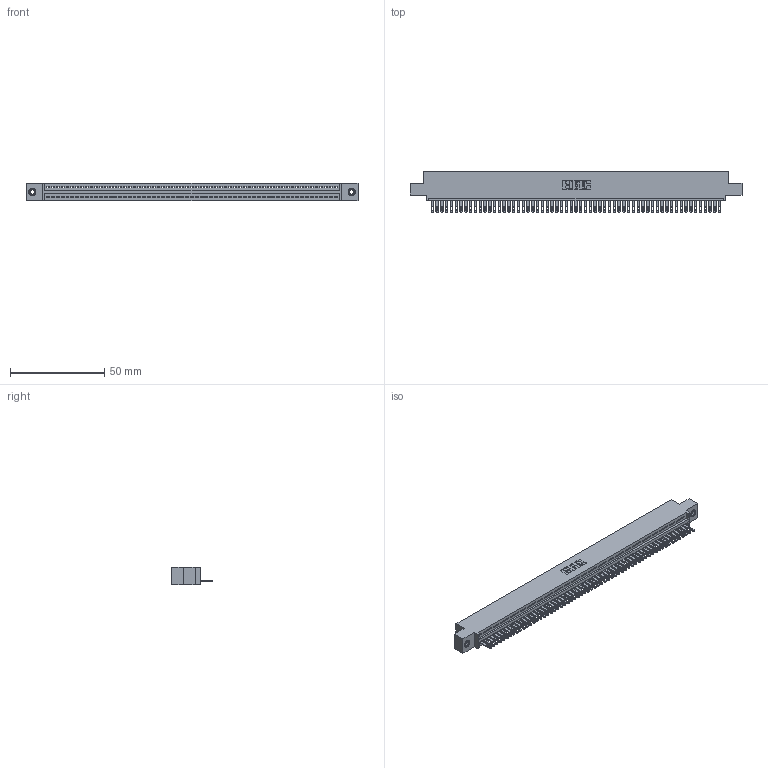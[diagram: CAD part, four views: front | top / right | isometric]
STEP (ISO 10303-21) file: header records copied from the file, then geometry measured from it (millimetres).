
FILE_DESCRIPTION (( 'STEP AP203' ), '1' );
FILE_NAME ('895-061-500-408.STEP', '2020-09-28T06:13:03', ( '' ), ( '' ), 'SwSTEP 2.0', 'SolidWorks 2020', '' );
FILE_SCHEMA (( 'CONFIG_CONTROL_DESIGN' ));
Length unit declared in the file: inch
Products named in the file (4): 345-292-001_345-293-100; 345-250-001_345-250-003-102; 895-061-500-408; 845 Part_0.110 Offset - 0.156 Dia-TI
Assembly tree (64 placements, depth 2):
  895-061-500-408
    845 Part_0.110 Offset - 0.156 Dia-TI
    345-292-001_345-293-100  x61
    345-250-001_345-250-003-102  x2
Bounding box: 176.15 x 21.51 x 9.4 mm (x, y, z)
Volume: 16844.3 mm3; surface area: 22880.8 mm2
Topology: 64 solids, 64 shells, 3484 faces, 10737 edges, 7150 vertices
Faces by surface type: plane 2190, cylinder 1278, cone 12, torus 4
Entity records: 44600 total; most frequent: CARTESIAN_POINT 7706, ORIENTED_EDGE 7694, DIRECTION 6731, EDGE_CURVE 3847, LINE 3447, VECTOR 3447, VERTEX_POINT 2560, AXIS2_PLACEMENT_3D 1642
